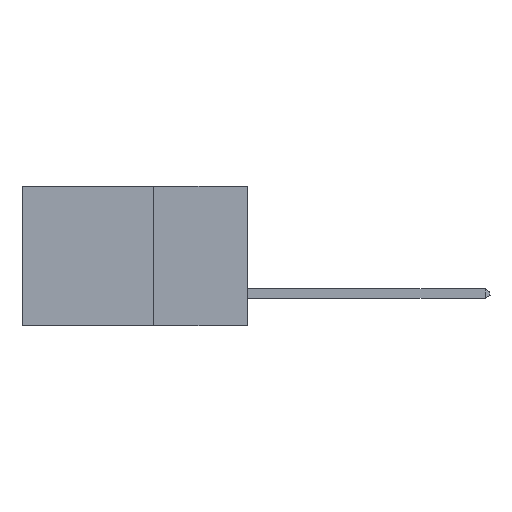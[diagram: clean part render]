
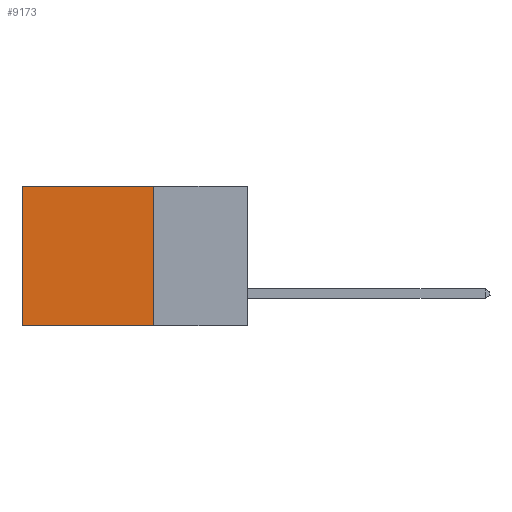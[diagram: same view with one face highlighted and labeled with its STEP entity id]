
A CAD part, left-side view. The second image highlights one B-rep face of the part: STEP entity #9173.
In plain terms, the highlighted planar face has unit normal (-1, 0, 0).
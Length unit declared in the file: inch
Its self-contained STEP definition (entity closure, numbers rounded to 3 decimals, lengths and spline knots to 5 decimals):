
#339 = CARTESIAN_POINT ( 'NONE',  ( 0.298, 0.25, 0. ) ) ;
#359 = VECTOR ( 'NONE', #13093, 39.37008 ) ;
#530 = ORIENTED_EDGE ( 'NONE', *, *, #7416, .F. ) ;
#657 = ORIENTED_EDGE ( 'NONE', *, *, #10887, .F. ) ;
#1208 = CARTESIAN_POINT ( 'NONE',  ( 0.298, 0.25, 0. ) ) ;
#1818 = CARTESIAN_POINT ( 'NONE',  ( 0.298, 0.25, 0. ) ) ;
#2795 = VERTEX_POINT ( 'NONE', #9982 ) ;
#2895 = VERTEX_POINT ( 'NONE', #11359 ) ;
#2954 = DIRECTION ( 'NONE',  ( 0., 0., -1. ) ) ;
#3432 = DIRECTION ( 'NONE',  ( 1., 0., 0. ) ) ;
#4495 = EDGE_LOOP ( 'NONE', ( #12873, #530, #657, #8707 ) ) ;
#4993 = VECTOR ( 'NONE', #7174, 39.37008 ) ;
#5806 = PLANE ( 'NONE',  #12839 ) ;
#6018 = CARTESIAN_POINT ( 'NONE',  ( 0.298, 0.6, 0. ) ) ;
#6820 = DIRECTION ( 'NONE',  ( 0., 0., -1. ) ) ;
#7174 = DIRECTION ( 'NONE',  ( 0., 1., 0. ) ) ;
#7416 = EDGE_CURVE ( 'NONE', #8884, #2795, #14274, .T. ) ;
#8079 = LINE ( 'NONE', #1208, #4993 ) ;
#8451 = LINE ( 'NONE', #1818, #12699 ) ;
#8649 = LINE ( 'NONE', #6018, #359 ) ;
#8707 = ORIENTED_EDGE ( 'NONE', *, *, #12562, .T. ) ;
#8884 = VERTEX_POINT ( 'NONE', #9826 ) ;
#9173 = ADVANCED_FACE ( 'NONE', ( #13099 ), #5806, .F. ) ;
#9826 = CARTESIAN_POINT ( 'NONE',  ( 0.298, 0.25, -0.37 ) ) ;
#9982 = CARTESIAN_POINT ( 'NONE',  ( 0.298, 0.6, -0.37 ) ) ;
#10273 = CARTESIAN_POINT ( 'NONE',  ( 0.298, 0.25, 0. ) ) ;
#10497 = CARTESIAN_POINT ( 'NONE',  ( 0.298, 0.25, -0.37 ) ) ;
#10887 = EDGE_CURVE ( 'NONE', #14557, #8884, #8451, .T. ) ;
#11359 = CARTESIAN_POINT ( 'NONE',  ( 0.298, 0.6, 0. ) ) ;
#11952 = EDGE_CURVE ( 'NONE', #2895, #2795, #8649, .T. ) ;
#12562 = EDGE_CURVE ( 'NONE', #14557, #2895, #8079, .T. ) ;
#12699 = VECTOR ( 'NONE', #2954, 39.37008 ) ;
#12839 = AXIS2_PLACEMENT_3D ( 'NONE', #10273, #3432, #6820 ) ;
#12873 = ORIENTED_EDGE ( 'NONE', *, *, #11952, .T. ) ;
#13093 = DIRECTION ( 'NONE',  ( 0., 0., -1. ) ) ;
#13099 = FACE_OUTER_BOUND ( 'NONE', #4495, .T. ) ;
#13553 = VECTOR ( 'NONE', #15214, 39.37008 ) ;
#14274 = LINE ( 'NONE', #10497, #13553 ) ;
#14557 = VERTEX_POINT ( 'NONE', #339 ) ;
#15214 = DIRECTION ( 'NONE',  ( 0., 1., 0. ) ) ;
